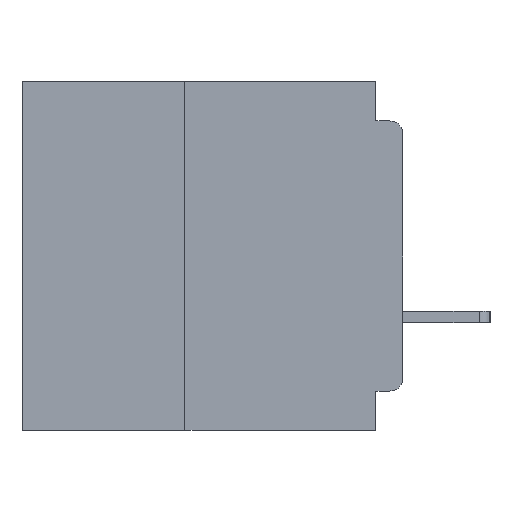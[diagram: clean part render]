
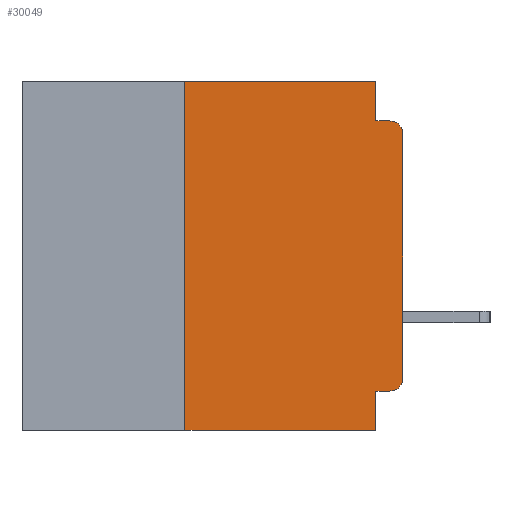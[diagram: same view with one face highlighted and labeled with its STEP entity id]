
A CAD part, left-side view. The second image highlights one B-rep face of the part: STEP entity #30049.
In plain terms, the highlighted planar face has unit normal (-1, 0, 0).
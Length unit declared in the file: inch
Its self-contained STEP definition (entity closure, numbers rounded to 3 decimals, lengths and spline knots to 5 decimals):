
#609 = VECTOR ( 'NONE', #35471, 39.37008 ) ;
#1506 = EDGE_CURVE ( 'NONE', #30591, #4781, #27355, .T. ) ;
#1569 = CARTESIAN_POINT ( 'NONE',  ( 0., 0.437, 0. ) ) ;
#2394 = LINE ( 'NONE', #19086, #609 ) ;
#2468 = DIRECTION ( 'NONE',  ( 0., 0., -1. ) ) ;
#4479 = DIRECTION ( 'NONE',  ( 0., 0., -1. ) ) ;
#4781 = VERTEX_POINT ( 'NONE', #25824 ) ;
#5109 = VECTOR ( 'NONE', #31988, 39.37008 ) ;
#5125 = AXIS2_PLACEMENT_3D ( 'NONE', #28306, #11794, #31066 ) ;
#5444 = VERTEX_POINT ( 'NONE', #12396 ) ;
#6623 = LINE ( 'NONE', #24040, #35159 ) ;
#6793 = VECTOR ( 'NONE', #27675, 39.37008 ) ;
#6973 = CARTESIAN_POINT ( 'NONE',  ( 0., 0.437, 0. ) ) ;
#7470 = ORIENTED_EDGE ( 'NONE', *, *, #9518, .F. ) ;
#7607 = ORIENTED_EDGE ( 'NONE', *, *, #19255, .F. ) ;
#7815 = ORIENTED_EDGE ( 'NONE', *, *, #1506, .F. ) ;
#8013 = VERTEX_POINT ( 'NONE', #11450 ) ;
#9320 = VERTEX_POINT ( 'NONE', #25600 ) ;
#9518 = EDGE_CURVE ( 'NONE', #8013, #30591, #23903, .T. ) ;
#9842 = CARTESIAN_POINT ( 'NONE',  ( 0., 0.25, -0.4 ) ) ;
#9891 = VERTEX_POINT ( 'NONE', #25074 ) ;
#10012 = EDGE_CURVE ( 'NONE', #9891, #19340, #2394, .T. ) ;
#10098 = LINE ( 'NONE', #29498, #30416 ) ;
#11450 = CARTESIAN_POINT ( 'NONE',  ( 0., 0.25, 0. ) ) ;
#11794 = DIRECTION ( 'NONE',  ( -1., 0., 0. ) ) ;
#12019 = AXIS2_PLACEMENT_3D ( 'NONE', #35716, #19332, #2468 ) ;
#12396 = CARTESIAN_POINT ( 'NONE',  ( 0., 0.015, -0.355 ) ) ;
#13514 = VECTOR ( 'NONE', #18327, 39.37008 ) ;
#13520 = LINE ( 'NONE', #9842, #26465 ) ;
#14818 = ORIENTED_EDGE ( 'NONE', *, *, #23957, .F. ) ;
#15462 = CARTESIAN_POINT ( 'NONE',  ( 0., 0., -0.045 ) ) ;
#15582 = EDGE_CURVE ( 'NONE', #9891, #8013, #13520, .T. ) ;
#15747 = DIRECTION ( 'NONE',  ( 0., 0., -1. ) ) ;
#15775 = DIRECTION ( 'NONE',  ( 0., 0., 1. ) ) ;
#16582 = VECTOR ( 'NONE', #26435, 39.37008 ) ;
#17060 = VERTEX_POINT ( 'NONE', #25622 ) ;
#17482 = EDGE_CURVE ( 'NONE', #26927, #9320, #19034, .T. ) ;
#18327 = DIRECTION ( 'NONE',  ( 0., -1., 0. ) ) ;
#18458 = PLANE ( 'NONE',  #33277 ) ;
#18799 = EDGE_CURVE ( 'NONE', #5444, #26960, #20672, .T. ) ;
#19034 = CIRCLE ( 'NONE', #12019, 0.015 ) ;
#19086 = CARTESIAN_POINT ( 'NONE',  ( 0., 0.437, -0.4 ) ) ;
#19255 = EDGE_CURVE ( 'NONE', #5444, #17060, #35315, .T. ) ;
#19332 = DIRECTION ( 'NONE',  ( -1., 0., 0. ) ) ;
#19340 = VERTEX_POINT ( 'NONE', #33487 ) ;
#20672 = CIRCLE ( 'NONE', #5125, 0.015 ) ;
#20865 = LINE ( 'NONE', #15462, #13514 ) ;
#21255 = DIRECTION ( 'NONE',  ( 1., 0., 0. ) ) ;
#21739 = ORIENTED_EDGE ( 'NONE', *, *, #22792, .T. ) ;
#22275 = FACE_OUTER_BOUND ( 'NONE', #25518, .T. ) ;
#22792 = EDGE_CURVE ( 'NONE', #26960, #26927, #10098, .T. ) ;
#23760 = DIRECTION ( 'NONE',  ( 0., 0., 1. ) ) ;
#23903 = LINE ( 'NONE', #6973, #16582 ) ;
#23957 = EDGE_CURVE ( 'NONE', #4781, #9320, #20865, .T. ) ;
#24040 = CARTESIAN_POINT ( 'NONE',  ( 0., 0.031, -0.4 ) ) ;
#24887 = CARTESIAN_POINT ( 'NONE',  ( 0., 0., -0.355 ) ) ;
#25026 = ORIENTED_EDGE ( 'NONE', *, *, #10012, .T. ) ;
#25074 = CARTESIAN_POINT ( 'NONE',  ( 0., 0.25, -0.4 ) ) ;
#25518 = EDGE_LOOP ( 'NONE', ( #21739, #34592, #14818, #7815, #7470, #31198, #25026, #32651, #7607, #25565 ) ) ;
#25565 = ORIENTED_EDGE ( 'NONE', *, *, #18799, .T. ) ;
#25600 = CARTESIAN_POINT ( 'NONE',  ( 0., 0.015, -0.045 ) ) ;
#25622 = CARTESIAN_POINT ( 'NONE',  ( 0., 0.031, -0.355 ) ) ;
#25824 = CARTESIAN_POINT ( 'NONE',  ( 0., 0.031, -0.045 ) ) ;
#26435 = DIRECTION ( 'NONE',  ( 0., -1., 0. ) ) ;
#26465 = VECTOR ( 'NONE', #23760, 39.37008 ) ;
#26927 = VERTEX_POINT ( 'NONE', #29623 ) ;
#26960 = VERTEX_POINT ( 'NONE', #32469 ) ;
#27355 = LINE ( 'NONE', #34693, #5109 ) ;
#27675 = DIRECTION ( 'NONE',  ( 0., 1., 0. ) ) ;
#28306 = CARTESIAN_POINT ( 'NONE',  ( 0., 0.015, -0.34 ) ) ;
#29274 = EDGE_CURVE ( 'NONE', #17060, #19340, #6623, .T. ) ;
#29498 = CARTESIAN_POINT ( 'NONE',  ( 0., 0., 0. ) ) ;
#29623 = CARTESIAN_POINT ( 'NONE',  ( 0., 0., -0.06 ) ) ;
#30049 = ADVANCED_FACE ( 'NONE', ( #22275 ), #18458, .F. ) ;
#30416 = VECTOR ( 'NONE', #15775, 39.37008 ) ;
#30591 = VERTEX_POINT ( 'NONE', #32124 ) ;
#31066 = DIRECTION ( 'NONE',  ( 0., 0., -1. ) ) ;
#31198 = ORIENTED_EDGE ( 'NONE', *, *, #15582, .F. ) ;
#31988 = DIRECTION ( 'NONE',  ( 0., 0., -1. ) ) ;
#32124 = CARTESIAN_POINT ( 'NONE',  ( 0., 0.031, 0. ) ) ;
#32469 = CARTESIAN_POINT ( 'NONE',  ( 0., 0., -0.34 ) ) ;
#32651 = ORIENTED_EDGE ( 'NONE', *, *, #29274, .F. ) ;
#33277 = AXIS2_PLACEMENT_3D ( 'NONE', #1569, #21255, #4479 ) ;
#33487 = CARTESIAN_POINT ( 'NONE',  ( 0., 0.031, -0.4 ) ) ;
#34592 = ORIENTED_EDGE ( 'NONE', *, *, #17482, .T. ) ;
#34693 = CARTESIAN_POINT ( 'NONE',  ( 0., 0.031, 0. ) ) ;
#35159 = VECTOR ( 'NONE', #15747, 39.37008 ) ;
#35315 = LINE ( 'NONE', #24887, #6793 ) ;
#35471 = DIRECTION ( 'NONE',  ( 0., -1., 0. ) ) ;
#35716 = CARTESIAN_POINT ( 'NONE',  ( 0., 0.015, -0.06 ) ) ;
